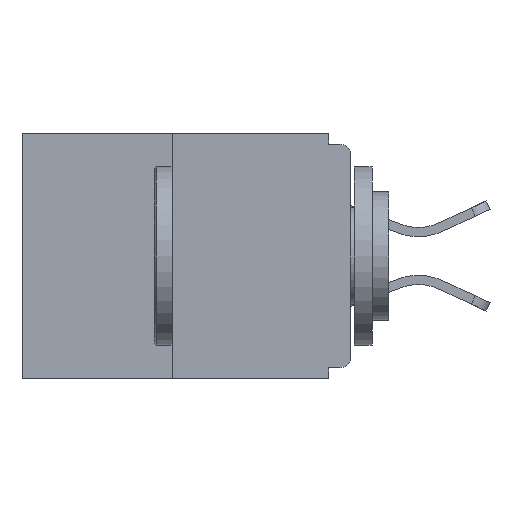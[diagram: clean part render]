
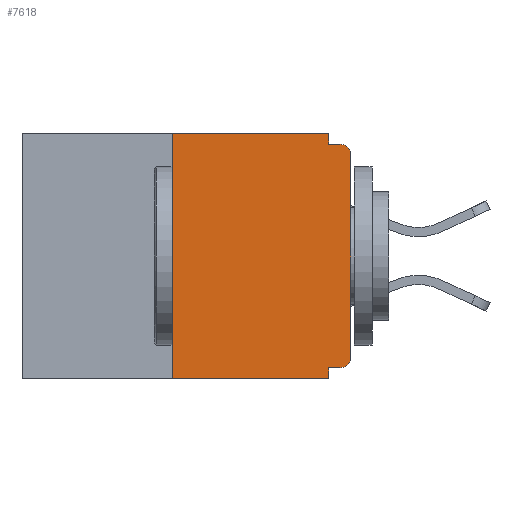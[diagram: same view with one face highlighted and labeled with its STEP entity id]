
A CAD part, left-side view. The second image highlights one B-rep face of the part: STEP entity #7618.
In plain terms, the highlighted planar face has unit normal (-1, 0, 0).
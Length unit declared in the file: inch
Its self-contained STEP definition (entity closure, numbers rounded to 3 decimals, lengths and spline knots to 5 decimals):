
#143 = FACE_OUTER_BOUND ( 'NONE', #3560, .T. ) ;
#199 = EDGE_CURVE ( 'NONE', #1401, #11820, #25367, .T. ) ;
#1401 = VERTEX_POINT ( 'NONE', #19816 ) ;
#2063 = ORIENTED_EDGE ( 'NONE', *, *, #3367, .F. ) ;
#2116 = AXIS2_PLACEMENT_3D ( 'NONE', #18354, #12128, #20191 ) ;
#2447 = VERTEX_POINT ( 'NONE', #22664 ) ;
#2667 = CIRCLE ( 'NONE', #25464, 0.015 ) ;
#2865 = DIRECTION ( 'NONE',  ( 0., -1., 0. ) ) ;
#3062 = CARTESIAN_POINT ( 'NONE',  ( 0., 0.46, -0.343 ) ) ;
#3178 = VERTEX_POINT ( 'NONE', #15125 ) ;
#3304 = PLANE ( 'NONE',  #2116 ) ;
#3367 = EDGE_CURVE ( 'NONE', #3178, #1401, #25492, .T. ) ;
#3560 = EDGE_LOOP ( 'NONE', ( #22988, #5467, #12834, #5510, #2063, #26038, #24902, #7476, #8926, #9544 ) ) ;
#3622 = LINE ( 'NONE', #3062, #23912 ) ;
#4202 = CIRCLE ( 'NONE', #24441, 0.015 ) ;
#5467 = ORIENTED_EDGE ( 'NONE', *, *, #17309, .F. ) ;
#5510 = ORIENTED_EDGE ( 'NONE', *, *, #199, .F. ) ;
#7476 = ORIENTED_EDGE ( 'NONE', *, *, #12491, .T. ) ;
#7618 = ADVANCED_FACE ( 'NONE', ( #143 ), #3304, .F. ) ;
#7695 = VECTOR ( 'NONE', #19106, 39.37008 ) ;
#7760 = DIRECTION ( 'NONE',  ( 0., 1., 0. ) ) ;
#7817 = EDGE_CURVE ( 'NONE', #17951, #15103, #11080, .T. ) ;
#8413 = DIRECTION ( 'NONE',  ( -1., 0., 0. ) ) ;
#8926 = ORIENTED_EDGE ( 'NONE', *, *, #25304, .F. ) ;
#9007 = LINE ( 'NONE', #14664, #7695 ) ;
#9329 = EDGE_CURVE ( 'NONE', #14169, #2447, #9007, .T. ) ;
#9485 = CARTESIAN_POINT ( 'NONE',  ( 0., 0.031, 0. ) ) ;
#9544 = ORIENTED_EDGE ( 'NONE', *, *, #27090, .F. ) ;
#9771 = EDGE_CURVE ( 'NONE', #3178, #17951, #2667, .T. ) ;
#10022 = LINE ( 'NONE', #25357, #19985 ) ;
#10574 = DIRECTION ( 'NONE',  ( 0., -1., 0. ) ) ;
#10953 = VECTOR ( 'NONE', #26210, 39.37008 ) ;
#11080 = LINE ( 'NONE', #25912, #11744 ) ;
#11224 = DIRECTION ( 'NONE',  ( 0., 0., 1. ) ) ;
#11744 = VECTOR ( 'NONE', #11224, 39.37008 ) ;
#11820 = VERTEX_POINT ( 'NONE', #14311 ) ;
#12128 = DIRECTION ( 'NONE',  ( 1., 0., 0. ) ) ;
#12433 = CARTESIAN_POINT ( 'NONE',  ( 0., 0.031, -0.343 ) ) ;
#12447 = CARTESIAN_POINT ( 'NONE',  ( 0., 0.25, 0. ) ) ;
#12491 = EDGE_CURVE ( 'NONE', #15103, #17779, #4202, .T. ) ;
#12834 = ORIENTED_EDGE ( 'NONE', *, *, #27547, .T. ) ;
#13084 = LINE ( 'NONE', #12447, #26388 ) ;
#13700 = VECTOR ( 'NONE', #14576, 39.37008 ) ;
#13789 = DIRECTION ( 'NONE',  ( 0., 0., -1. ) ) ;
#14169 = VERTEX_POINT ( 'NONE', #23321 ) ;
#14188 = VECTOR ( 'NONE', #7760, 39.37008 ) ;
#14311 = CARTESIAN_POINT ( 'NONE',  ( 0., 0.031, -0.343 ) ) ;
#14576 = DIRECTION ( 'NONE',  ( 0., 0., -1. ) ) ;
#14664 = CARTESIAN_POINT ( 'NONE',  ( 0., 0.46, 0. ) ) ;
#15103 = VERTEX_POINT ( 'NONE', #23470 ) ;
#15125 = CARTESIAN_POINT ( 'NONE',  ( 0., 0.015, -0.328 ) ) ;
#16013 = VERTEX_POINT ( 'NONE', #20246 ) ;
#17309 = EDGE_CURVE ( 'NONE', #23841, #14169, #13084, .T. ) ;
#17779 = VERTEX_POINT ( 'NONE', #23794 ) ;
#17951 = VERTEX_POINT ( 'NONE', #20143 ) ;
#18354 = CARTESIAN_POINT ( 'NONE',  ( 0., 0.46, 0. ) ) ;
#18977 = CARTESIAN_POINT ( 'NONE',  ( 0., 0.015, -0.03 ) ) ;
#19106 = DIRECTION ( 'NONE',  ( 0., -1., 0. ) ) ;
#19816 = CARTESIAN_POINT ( 'NONE',  ( 0., 0.031, -0.328 ) ) ;
#19985 = VECTOR ( 'NONE', #10574, 39.37008 ) ;
#20082 = CARTESIAN_POINT ( 'NONE',  ( 0., 0.015, -0.313 ) ) ;
#20098 = CARTESIAN_POINT ( 'NONE',  ( 0., 0.25, -0.343 ) ) ;
#20143 = CARTESIAN_POINT ( 'NONE',  ( 0., 0., -0.313 ) ) ;
#20191 = DIRECTION ( 'NONE',  ( 0., 0., -1. ) ) ;
#20246 = CARTESIAN_POINT ( 'NONE',  ( 0., 0.031, -0.015 ) ) ;
#20580 = LINE ( 'NONE', #9485, #10953 ) ;
#22664 = CARTESIAN_POINT ( 'NONE',  ( 0., 0.031, 0. ) ) ;
#22694 = CARTESIAN_POINT ( 'NONE',  ( 0., 0., -0.328 ) ) ;
#22988 = ORIENTED_EDGE ( 'NONE', *, *, #9329, .F. ) ;
#23321 = CARTESIAN_POINT ( 'NONE',  ( 0., 0.25, 0. ) ) ;
#23433 = DIRECTION ( 'NONE',  ( 0., 0., -1. ) ) ;
#23470 = CARTESIAN_POINT ( 'NONE',  ( 0., 0., -0.03 ) ) ;
#23794 = CARTESIAN_POINT ( 'NONE',  ( 0., 0.015, -0.015 ) ) ;
#23841 = VERTEX_POINT ( 'NONE', #20098 ) ;
#23912 = VECTOR ( 'NONE', #2865, 39.37008 ) ;
#24441 = AXIS2_PLACEMENT_3D ( 'NONE', #18977, #8413, #23433 ) ;
#24902 = ORIENTED_EDGE ( 'NONE', *, *, #7817, .T. ) ;
#25304 = EDGE_CURVE ( 'NONE', #16013, #17779, #10022, .T. ) ;
#25357 = CARTESIAN_POINT ( 'NONE',  ( 0., 0., -0.015 ) ) ;
#25367 = LINE ( 'NONE', #12433, #13700 ) ;
#25464 = AXIS2_PLACEMENT_3D ( 'NONE', #20082, #26521, #13789 ) ;
#25492 = LINE ( 'NONE', #22694, #14188 ) ;
#25912 = CARTESIAN_POINT ( 'NONE',  ( 0., 0., 0. ) ) ;
#26038 = ORIENTED_EDGE ( 'NONE', *, *, #9771, .T. ) ;
#26210 = DIRECTION ( 'NONE',  ( 0., 0., -1. ) ) ;
#26388 = VECTOR ( 'NONE', #27490, 39.37008 ) ;
#26521 = DIRECTION ( 'NONE',  ( -1., 0., 0. ) ) ;
#27090 = EDGE_CURVE ( 'NONE', #2447, #16013, #20580, .T. ) ;
#27490 = DIRECTION ( 'NONE',  ( 0., 0., 1. ) ) ;
#27547 = EDGE_CURVE ( 'NONE', #23841, #11820, #3622, .T. ) ;
